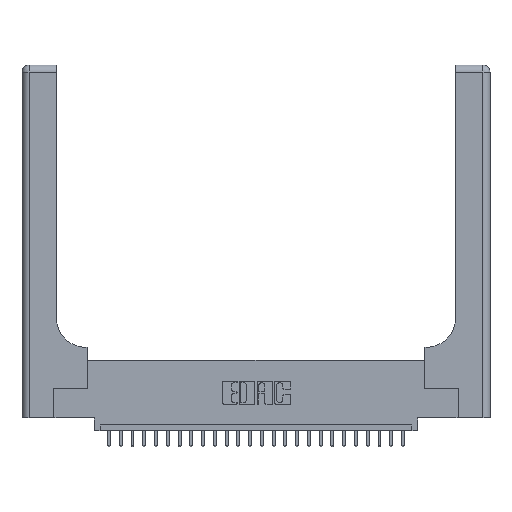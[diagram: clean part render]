
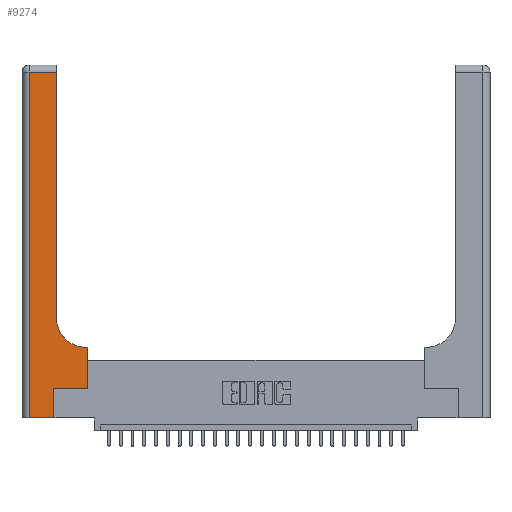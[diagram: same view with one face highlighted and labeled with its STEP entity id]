
A CAD part, top view. The second image highlights one B-rep face of the part: STEP entity #9274.
In plain terms, the highlighted planar face has unit normal (0, 0, 1).
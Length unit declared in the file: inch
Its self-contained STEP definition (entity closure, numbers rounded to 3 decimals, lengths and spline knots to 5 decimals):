
#167 = CARTESIAN_POINT ( 'NONE',  ( 0., 0., 0.37 ) ) ;
#446 = VECTOR ( 'NONE', #8230, 39.37008 ) ;
#683 = LINE ( 'NONE', #2566, #17997 ) ;
#811 = CARTESIAN_POINT ( 'NONE',  ( 0.269, 0., 0.37 ) ) ;
#986 = VERTEX_POINT ( 'NONE', #10310 ) ;
#1448 = CARTESIAN_POINT ( 'NONE',  ( 0.5585, 0.6, 0.37 ) ) ;
#1748 = VERTEX_POINT ( 'NONE', #9909 ) ;
#2217 = VECTOR ( 'NONE', #15054, 39.37008 ) ;
#2366 = LINE ( 'NONE', #167, #12836 ) ;
#2369 = VERTEX_POINT ( 'NONE', #9082 ) ;
#2566 = CARTESIAN_POINT ( 'NONE',  ( 0., 2.94, 0.37 ) ) ;
#2784 = VERTEX_POINT ( 'NONE', #10043 ) ;
#2837 = CARTESIAN_POINT ( 'NONE',  ( 0.2915, 3., 0.37 ) ) ;
#3036 = VERTEX_POINT ( 'NONE', #1448 ) ;
#3037 = ORIENTED_EDGE ( 'NONE', *, *, #4142, .T. ) ;
#3333 = LINE ( 'NONE', #19480, #22261 ) ;
#3495 = ORIENTED_EDGE ( 'NONE', *, *, #15335, .T. ) ;
#3588 = EDGE_CURVE ( 'NONE', #2369, #986, #24740, .T. ) ;
#4142 = EDGE_CURVE ( 'NONE', #5820, #3036, #25040, .T. ) ;
#4197 = ORIENTED_EDGE ( 'NONE', *, *, #19385, .T. ) ;
#4648 = DIRECTION ( 'NONE',  ( -1., 0., 0. ) ) ;
#5604 = DIRECTION ( 'NONE',  ( 0., 0., -1. ) ) ;
#5820 = VERTEX_POINT ( 'NONE', #26962 ) ;
#6011 = VECTOR ( 'NONE', #4648, 39.37008 ) ;
#6125 = CARTESIAN_POINT ( 'NONE',  ( 0.269, 0.25, 0.37 ) ) ;
#6485 = VECTOR ( 'NONE', #6648, 39.37008 ) ;
#6648 = DIRECTION ( 'NONE',  ( 0., 1., 0. ) ) ;
#7026 = DIRECTION ( 'NONE',  ( 0., 1., 0. ) ) ;
#7327 = ORIENTED_EDGE ( 'NONE', *, *, #3588, .T. ) ;
#7705 = VERTEX_POINT ( 'NONE', #15843 ) ;
#8001 = ORIENTED_EDGE ( 'NONE', *, *, #15370, .T. ) ;
#8104 = ORIENTED_EDGE ( 'NONE', *, *, #25578, .T. ) ;
#8230 = DIRECTION ( 'NONE',  ( 1., 0., 0. ) ) ;
#8743 = CARTESIAN_POINT ( 'NONE',  ( 0.2915, 0.6, 0.37 ) ) ;
#8861 = CARTESIAN_POINT ( 'NONE',  ( 0.5585, 0.25, 0.37 ) ) ;
#9082 = CARTESIAN_POINT ( 'NONE',  ( 0.2915, 0.85, 0.37 ) ) ;
#9274 = ADVANCED_FACE ( 'NONE', ( #12802 ), #23376, .F. ) ;
#9909 = CARTESIAN_POINT ( 'NONE',  ( 0.06, 2.94, 0.37 ) ) ;
#10043 = CARTESIAN_POINT ( 'NONE',  ( 0.06, 0., 0.37 ) ) ;
#10310 = CARTESIAN_POINT ( 'NONE',  ( 0.2915, 2.94, 0.37 ) ) ;
#11503 = CARTESIAN_POINT ( 'NONE',  ( 0.5415, 0.85, 0.37 ) ) ;
#11892 = LINE ( 'NONE', #6125, #446 ) ;
#12802 = FACE_OUTER_BOUND ( 'NONE', #20589, .T. ) ;
#12836 = VECTOR ( 'NONE', #18980, 39.37008 ) ;
#13382 = DIRECTION ( 'NONE',  ( 0., -1., 0. ) ) ;
#14190 = LINE ( 'NONE', #8743, #6011 ) ;
#14713 = EDGE_CURVE ( 'NONE', #2784, #7705, #2366, .T. ) ;
#15054 = DIRECTION ( 'NONE',  ( 0., 1., 0. ) ) ;
#15184 = VERTEX_POINT ( 'NONE', #23568 ) ;
#15335 = EDGE_CURVE ( 'NONE', #1748, #2784, #3333, .T. ) ;
#15370 = EDGE_CURVE ( 'NONE', #986, #1748, #683, .T. ) ;
#15391 = AXIS2_PLACEMENT_3D ( 'NONE', #11503, #5604, #26424 ) ;
#15462 = CIRCLE ( 'NONE', #15391, 0.25 ) ;
#15813 = VECTOR ( 'NONE', #7026, 39.37008 ) ;
#15843 = CARTESIAN_POINT ( 'NONE',  ( 0.269, 0., 0.37 ) ) ;
#15952 = AXIS2_PLACEMENT_3D ( 'NONE', #26876, #17282, #16636 ) ;
#16636 = DIRECTION ( 'NONE',  ( -1., 0., 0. ) ) ;
#16782 = ORIENTED_EDGE ( 'NONE', *, *, #14713, .T. ) ;
#17150 = DIRECTION ( 'NONE',  ( -1., 0., 0. ) ) ;
#17282 = DIRECTION ( 'NONE',  ( 0., 0., -1. ) ) ;
#17487 = VERTEX_POINT ( 'NONE', #26251 ) ;
#17997 = VECTOR ( 'NONE', #17150, 39.37008 ) ;
#18980 = DIRECTION ( 'NONE',  ( 1., 0., 0. ) ) ;
#19385 = EDGE_CURVE ( 'NONE', #17487, #2369, #15462, .T. ) ;
#19480 = CARTESIAN_POINT ( 'NONE',  ( 0.06, 3., 0.37 ) ) ;
#19541 = ORIENTED_EDGE ( 'NONE', *, *, #26255, .T. ) ;
#20589 = EDGE_LOOP ( 'NONE', ( #7327, #8001, #3495, #16782, #8104, #19541, #3037, #23873, #4197 ) ) ;
#21389 = LINE ( 'NONE', #811, #15813 ) ;
#22261 = VECTOR ( 'NONE', #13382, 39.37008 ) ;
#23376 = PLANE ( 'NONE',  #15952 ) ;
#23568 = CARTESIAN_POINT ( 'NONE',  ( 0.269, 0.25, 0.37 ) ) ;
#23873 = ORIENTED_EDGE ( 'NONE', *, *, #25475, .T. ) ;
#24740 = LINE ( 'NONE', #2837, #6485 ) ;
#25040 = LINE ( 'NONE', #8861, #2217 ) ;
#25475 = EDGE_CURVE ( 'NONE', #3036, #17487, #14190, .T. ) ;
#25578 = EDGE_CURVE ( 'NONE', #7705, #15184, #21389, .T. ) ;
#26251 = CARTESIAN_POINT ( 'NONE',  ( 0.5415, 0.6, 0.37 ) ) ;
#26255 = EDGE_CURVE ( 'NONE', #15184, #5820, #11892, .T. ) ;
#26424 = DIRECTION ( 'NONE',  ( 1., 0., 0. ) ) ;
#26876 = CARTESIAN_POINT ( 'NONE',  ( 0., 3., 0.37 ) ) ;
#26962 = CARTESIAN_POINT ( 'NONE',  ( 0.5585, 0.25, 0.37 ) ) ;
